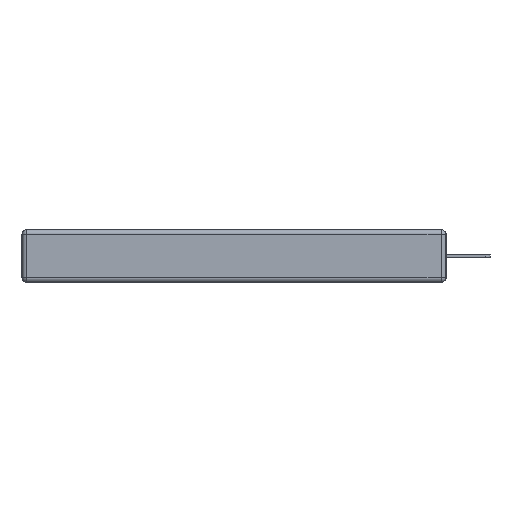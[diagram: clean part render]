
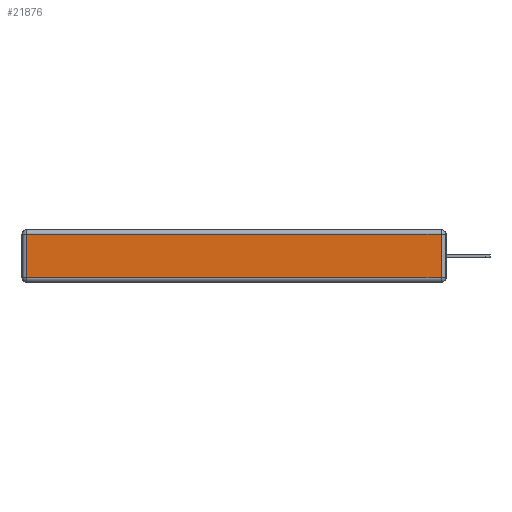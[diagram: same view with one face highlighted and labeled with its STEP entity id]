
A CAD part, left-side view. The second image highlights one B-rep face of the part: STEP entity #21876.
In plain terms, the highlighted planar face has unit normal (-1, 0, 0).
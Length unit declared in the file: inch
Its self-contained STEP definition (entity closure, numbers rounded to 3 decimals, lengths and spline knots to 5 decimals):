
#2049 = DIRECTION ( 'NONE',  ( 0., -1., 0. ) ) ;
#2588 = CARTESIAN_POINT ( 'NONE',  ( 0., 0.03, -0.313 ) ) ;
#3435 = LINE ( 'NONE', #21764, #21735 ) ;
#3667 = VERTEX_POINT ( 'NONE', #10539 ) ;
#4499 = CARTESIAN_POINT ( 'NONE',  ( 0., 2.72, -0.313 ) ) ;
#5741 = EDGE_CURVE ( 'NONE', #8688, #22744, #10254, .T. ) ;
#5773 = DIRECTION ( 'NONE',  ( -1., 0., 0. ) ) ;
#5866 = ORIENTED_EDGE ( 'NONE', *, *, #5741, .T. ) ;
#5881 = ORIENTED_EDGE ( 'NONE', *, *, #20992, .T. ) ;
#6366 = CARTESIAN_POINT ( 'NONE',  ( 0., 2.75, -0.03 ) ) ;
#7268 = FACE_OUTER_BOUND ( 'NONE', #14344, .T. ) ;
#8090 = LINE ( 'NONE', #6366, #11569 ) ;
#8176 = EDGE_CURVE ( 'NONE', #3667, #20139, #8090, .T. ) ;
#8533 = VECTOR ( 'NONE', #2049, 39.37008 ) ;
#8688 = VERTEX_POINT ( 'NONE', #4499 ) ;
#9946 = ORIENTED_EDGE ( 'NONE', *, *, #10672, .T. ) ;
#10254 = LINE ( 'NONE', #17286, #8533 ) ;
#10539 = CARTESIAN_POINT ( 'NONE',  ( 0., 0.03, -0.03 ) ) ;
#10672 = EDGE_CURVE ( 'NONE', #20139, #8688, #14523, .T. ) ;
#11569 = VECTOR ( 'NONE', #20468, 39.37008 ) ;
#12460 = DIRECTION ( 'NONE',  ( 0., 0., 1. ) ) ;
#14181 = VECTOR ( 'NONE', #16457, 39.37008 ) ;
#14344 = EDGE_LOOP ( 'NONE', ( #5866, #5881, #15103, #9946 ) ) ;
#14523 = LINE ( 'NONE', #16126, #14181 ) ;
#15103 = ORIENTED_EDGE ( 'NONE', *, *, #8176, .T. ) ;
#16126 = CARTESIAN_POINT ( 'NONE',  ( 0., 2.72, -0.343 ) ) ;
#16243 = AXIS2_PLACEMENT_3D ( 'NONE', #17802, #5773, #21712 ) ;
#16457 = DIRECTION ( 'NONE',  ( 0., 0., -1. ) ) ;
#17286 = CARTESIAN_POINT ( 'NONE',  ( 0., 0., -0.313 ) ) ;
#17802 = CARTESIAN_POINT ( 'NONE',  ( 0., 0., -0.343 ) ) ;
#18026 = PLANE ( 'NONE',  #16243 ) ;
#19319 = CARTESIAN_POINT ( 'NONE',  ( 0., 2.72, -0.03 ) ) ;
#20139 = VERTEX_POINT ( 'NONE', #19319 ) ;
#20468 = DIRECTION ( 'NONE',  ( 0., 1., 0. ) ) ;
#20992 = EDGE_CURVE ( 'NONE', #22744, #3667, #3435, .T. ) ;
#21712 = DIRECTION ( 'NONE',  ( 0., 0., 1. ) ) ;
#21735 = VECTOR ( 'NONE', #12460, 39.37008 ) ;
#21764 = CARTESIAN_POINT ( 'NONE',  ( 0., 0.03, -0.343 ) ) ;
#21876 = ADVANCED_FACE ( 'NONE', ( #7268 ), #18026, .T. ) ;
#22744 = VERTEX_POINT ( 'NONE', #2588 ) ;
